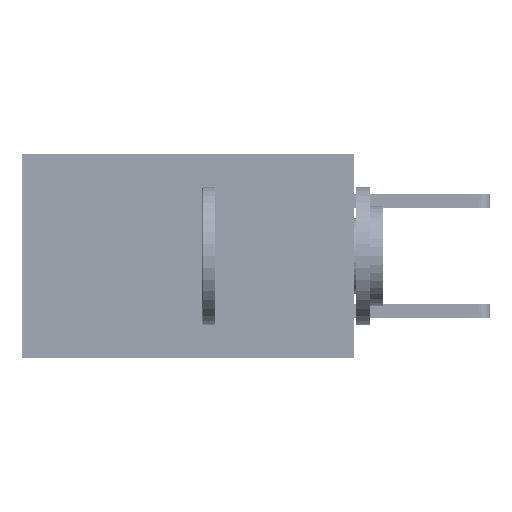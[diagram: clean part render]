
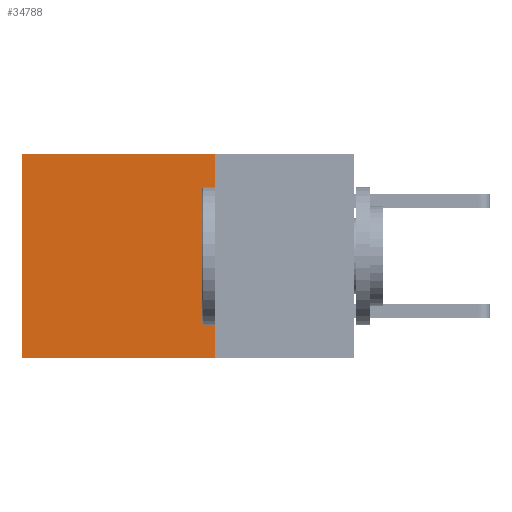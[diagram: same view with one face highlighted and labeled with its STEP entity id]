
A CAD part, left-side view. The second image highlights one B-rep face of the part: STEP entity #34788.
In plain terms, the highlighted planar face has unit normal (-1, 0, 0).
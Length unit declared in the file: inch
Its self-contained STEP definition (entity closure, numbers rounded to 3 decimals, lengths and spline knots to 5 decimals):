
#509 = ORIENTED_EDGE ( 'NONE', *, *, #30454, .T. ) ;
#4400 = AXIS2_PLACEMENT_3D ( 'NONE', #23553, #4485, #39484 ) ;
#4485 = DIRECTION ( 'NONE',  ( 1., 0., 0. ) ) ;
#4783 = DIRECTION ( 'NONE',  ( 0., 1., 0. ) ) ;
#5456 = VECTOR ( 'NONE', #15451, 39.37008 ) ;
#5879 = EDGE_CURVE ( 'NONE', #32645, #7872, #22313, .T. ) ;
#7872 = VERTEX_POINT ( 'NONE', #16196 ) ;
#9446 = EDGE_LOOP ( 'NONE', ( #33715, #30162, #33787, #509 ) ) ;
#9752 = VERTEX_POINT ( 'NONE', #35244 ) ;
#12516 = VECTOR ( 'NONE', #16452, 39.37008 ) ;
#13813 = LINE ( 'NONE', #21508, #5456 ) ;
#14088 = PLANE ( 'NONE',  #4400 ) ;
#15451 = DIRECTION ( 'NONE',  ( 0., 0., -1. ) ) ;
#15971 = CARTESIAN_POINT ( 'NONE',  ( 0.2875, 0.6, 0. ) ) ;
#16196 = CARTESIAN_POINT ( 'NONE',  ( 0.2875, 0.6, -0.37 ) ) ;
#16278 = EDGE_CURVE ( 'NONE', #9752, #32645, #13813, .T. ) ;
#16452 = DIRECTION ( 'NONE',  ( 0., 1., 0. ) ) ;
#17024 = CARTESIAN_POINT ( 'NONE',  ( 0.2875, 0.6, 0. ) ) ;
#17654 = CARTESIAN_POINT ( 'NONE',  ( 0.2875, 0.25, 0. ) ) ;
#21508 = CARTESIAN_POINT ( 'NONE',  ( 0.2875, 0.25, 0. ) ) ;
#22313 = LINE ( 'NONE', #30970, #12516 ) ;
#22721 = FACE_OUTER_BOUND ( 'NONE', #9446, .T. ) ;
#23553 = CARTESIAN_POINT ( 'NONE',  ( 0.2875, 0.25, 0. ) ) ;
#24534 = LINE ( 'NONE', #17654, #31360 ) ;
#28416 = LINE ( 'NONE', #17024, #34802 ) ;
#30035 = DIRECTION ( 'NONE',  ( 0., 0., -1. ) ) ;
#30162 = ORIENTED_EDGE ( 'NONE', *, *, #5879, .F. ) ;
#30454 = EDGE_CURVE ( 'NONE', #9752, #34504, #24534, .T. ) ;
#30970 = CARTESIAN_POINT ( 'NONE',  ( 0.2875, 0.25, -0.37 ) ) ;
#31360 = VECTOR ( 'NONE', #4783, 39.37008 ) ;
#32645 = VERTEX_POINT ( 'NONE', #35008 ) ;
#33715 = ORIENTED_EDGE ( 'NONE', *, *, #36793, .T. ) ;
#33787 = ORIENTED_EDGE ( 'NONE', *, *, #16278, .F. ) ;
#34504 = VERTEX_POINT ( 'NONE', #15971 ) ;
#34788 = ADVANCED_FACE ( 'NONE', ( #22721 ), #14088, .F. ) ;
#34802 = VECTOR ( 'NONE', #30035, 39.37008 ) ;
#35008 = CARTESIAN_POINT ( 'NONE',  ( 0.2875, 0.25, -0.37 ) ) ;
#35244 = CARTESIAN_POINT ( 'NONE',  ( 0.2875, 0.25, 0. ) ) ;
#36793 = EDGE_CURVE ( 'NONE', #34504, #7872, #28416, .T. ) ;
#39484 = DIRECTION ( 'NONE',  ( 0., 0., -1. ) ) ;
